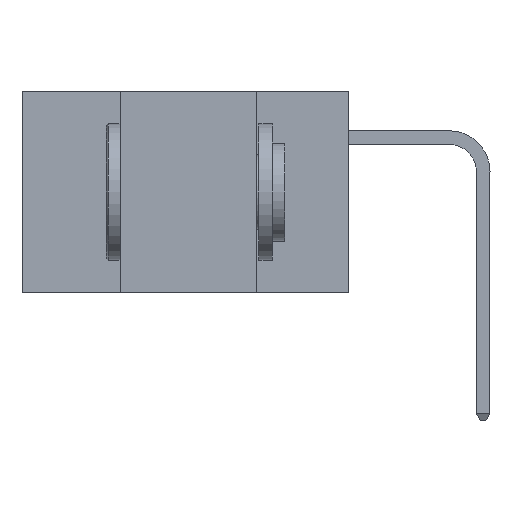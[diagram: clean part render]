
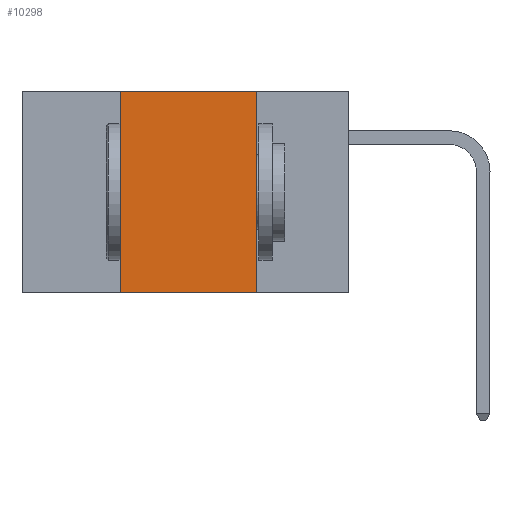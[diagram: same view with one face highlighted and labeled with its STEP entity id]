
A CAD part, left-side view. The second image highlights one B-rep face of the part: STEP entity #10298.
In plain terms, the highlighted planar face has unit normal (-1, 0, 0).
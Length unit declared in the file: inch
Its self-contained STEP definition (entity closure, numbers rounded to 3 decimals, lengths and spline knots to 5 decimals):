
#581 = VECTOR ( 'NONE', #19962, 39.37008 ) ;
#1914 = FACE_OUTER_BOUND ( 'NONE', #9162, .T. ) ;
#4280 = VERTEX_POINT ( 'NONE', #22210 ) ;
#4684 = CARTESIAN_POINT ( 'NONE',  ( 0., 0.6, 0. ) ) ;
#6930 = EDGE_CURVE ( 'NONE', #4280, #24561, #36656, .T. ) ;
#8864 = EDGE_CURVE ( 'NONE', #24992, #26395, #11459, .T. ) ;
#9101 = EDGE_CURVE ( 'NONE', #24992, #24561, #23527, .T. ) ;
#9162 = EDGE_LOOP ( 'NONE', ( #20534, #30793, #18412, #36995 ) ) ;
#9943 = VECTOR ( 'NONE', #27599, 39.37008 ) ;
#10298 = ADVANCED_FACE ( 'NONE', ( #1914 ), #11489, .F. ) ;
#10827 = LINE ( 'NONE', #4684, #9943 ) ;
#11459 = LINE ( 'NONE', #35699, #18221 ) ;
#11489 = PLANE ( 'NONE',  #29971 ) ;
#11590 = EDGE_CURVE ( 'NONE', #26395, #4280, #10827, .T. ) ;
#12153 = CARTESIAN_POINT ( 'NONE',  ( 0., 0.42, 0. ) ) ;
#12278 = CARTESIAN_POINT ( 'NONE',  ( 0., 0.17, -0.37 ) ) ;
#13987 = VECTOR ( 'NONE', #19893, 39.37008 ) ;
#14348 = DIRECTION ( 'NONE',  ( 0., 0., -1. ) ) ;
#17104 = CARTESIAN_POINT ( 'NONE',  ( 0., 0.6, -0.37 ) ) ;
#18221 = VECTOR ( 'NONE', #24488, 39.37008 ) ;
#18412 = ORIENTED_EDGE ( 'NONE', *, *, #8864, .F. ) ;
#19776 = CARTESIAN_POINT ( 'NONE',  ( 0., 0.17, 0. ) ) ;
#19893 = DIRECTION ( 'NONE',  ( 0., 0., -1. ) ) ;
#19962 = DIRECTION ( 'NONE',  ( 0., -1., 0. ) ) ;
#20534 = ORIENTED_EDGE ( 'NONE', *, *, #6930, .F. ) ;
#22210 = CARTESIAN_POINT ( 'NONE',  ( 0., 0.17, 0. ) ) ;
#22956 = CARTESIAN_POINT ( 'NONE',  ( 0., 0.42, -0.37 ) ) ;
#23527 = LINE ( 'NONE', #17104, #581 ) ;
#24488 = DIRECTION ( 'NONE',  ( 0., 0., 1. ) ) ;
#24561 = VERTEX_POINT ( 'NONE', #12278 ) ;
#24992 = VERTEX_POINT ( 'NONE', #22956 ) ;
#26395 = VERTEX_POINT ( 'NONE', #12153 ) ;
#27599 = DIRECTION ( 'NONE',  ( 0., -1., 0. ) ) ;
#28604 = CARTESIAN_POINT ( 'NONE',  ( 0., 0.6, 0. ) ) ;
#29971 = AXIS2_PLACEMENT_3D ( 'NONE', #28604, #31437, #14348 ) ;
#30793 = ORIENTED_EDGE ( 'NONE', *, *, #11590, .F. ) ;
#31437 = DIRECTION ( 'NONE',  ( 1., 0., 0. ) ) ;
#35699 = CARTESIAN_POINT ( 'NONE',  ( 0., 0.42, 0. ) ) ;
#36656 = LINE ( 'NONE', #19776, #13987 ) ;
#36995 = ORIENTED_EDGE ( 'NONE', *, *, #9101, .T. ) ;
